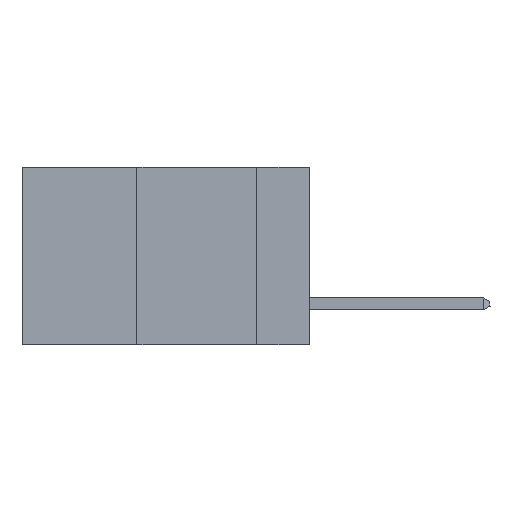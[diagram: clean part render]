
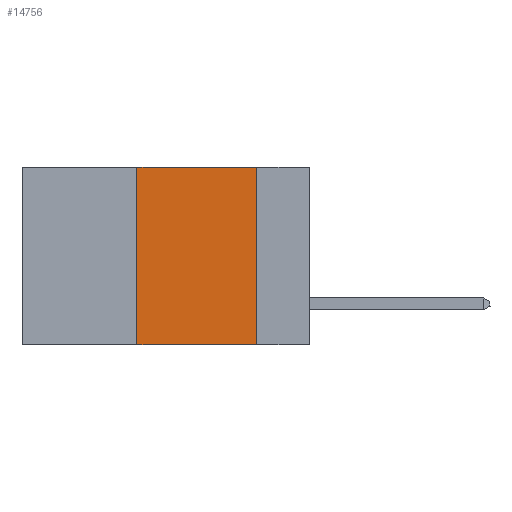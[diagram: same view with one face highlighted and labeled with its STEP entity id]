
A CAD part, left-side view. The second image highlights one B-rep face of the part: STEP entity #14756.
In plain terms, the highlighted planar face has unit normal (-1, 0, 0).
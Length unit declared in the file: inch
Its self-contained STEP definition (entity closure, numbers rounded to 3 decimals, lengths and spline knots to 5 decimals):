
#131 = LINE ( 'NONE', #13312, #3278 ) ;
#155 = EDGE_LOOP ( 'NONE', ( #30151, #12103, #18342, #29159 ) ) ;
#494 = CARTESIAN_POINT ( 'NONE',  ( 0., 0.6, 0. ) ) ;
#620 = VERTEX_POINT ( 'NONE', #14677 ) ;
#625 = DIRECTION ( 'NONE',  ( 0., -1., 0. ) ) ;
#1336 = DIRECTION ( 'NONE',  ( 0., -1., 0. ) ) ;
#3077 = VERTEX_POINT ( 'NONE', #8874 ) ;
#3278 = VECTOR ( 'NONE', #1336, 39.37008 ) ;
#4525 = DIRECTION ( 'NONE',  ( 0., 0., -1. ) ) ;
#6027 = CARTESIAN_POINT ( 'NONE',  ( 0., 0.36, -0.37 ) ) ;
#6850 = AXIS2_PLACEMENT_3D ( 'NONE', #14929, #17680, #15182 ) ;
#8874 = CARTESIAN_POINT ( 'NONE',  ( 0., 0.36, 0. ) ) ;
#12103 = ORIENTED_EDGE ( 'NONE', *, *, #35129, .F. ) ;
#12367 = VECTOR ( 'NONE', #25544, 39.37008 ) ;
#13312 = CARTESIAN_POINT ( 'NONE',  ( 0., 0.6, -0.37 ) ) ;
#13877 = EDGE_CURVE ( 'NONE', #620, #34804, #23092, .T. ) ;
#14677 = CARTESIAN_POINT ( 'NONE',  ( 0., 0.11, 0. ) ) ;
#14756 = ADVANCED_FACE ( 'NONE', ( #32384 ), #34950, .F. ) ;
#14929 = CARTESIAN_POINT ( 'NONE',  ( 0., 0.6, 0. ) ) ;
#15182 = DIRECTION ( 'NONE',  ( 0., 0., -1. ) ) ;
#17680 = DIRECTION ( 'NONE',  ( 1., 0., 0. ) ) ;
#18342 = ORIENTED_EDGE ( 'NONE', *, *, #24578, .F. ) ;
#19098 = VECTOR ( 'NONE', #625, 39.37008 ) ;
#23092 = LINE ( 'NONE', #24269, #24443 ) ;
#24269 = CARTESIAN_POINT ( 'NONE',  ( 0., 0.11, 0. ) ) ;
#24443 = VECTOR ( 'NONE', #4525, 39.37008 ) ;
#24578 = EDGE_CURVE ( 'NONE', #35182, #3077, #35308, .T. ) ;
#25544 = DIRECTION ( 'NONE',  ( 0., 0., 1. ) ) ;
#27173 = LINE ( 'NONE', #494, #19098 ) ;
#29159 = ORIENTED_EDGE ( 'NONE', *, *, #37118, .T. ) ;
#30151 = ORIENTED_EDGE ( 'NONE', *, *, #13877, .F. ) ;
#30724 = CARTESIAN_POINT ( 'NONE',  ( 0., 0.36, 0. ) ) ;
#32384 = FACE_OUTER_BOUND ( 'NONE', #155, .T. ) ;
#33602 = CARTESIAN_POINT ( 'NONE',  ( 0., 0.11, -0.37 ) ) ;
#34804 = VERTEX_POINT ( 'NONE', #33602 ) ;
#34950 = PLANE ( 'NONE',  #6850 ) ;
#35129 = EDGE_CURVE ( 'NONE', #3077, #620, #27173, .T. ) ;
#35182 = VERTEX_POINT ( 'NONE', #6027 ) ;
#35308 = LINE ( 'NONE', #30724, #12367 ) ;
#37118 = EDGE_CURVE ( 'NONE', #35182, #34804, #131, .T. ) ;
